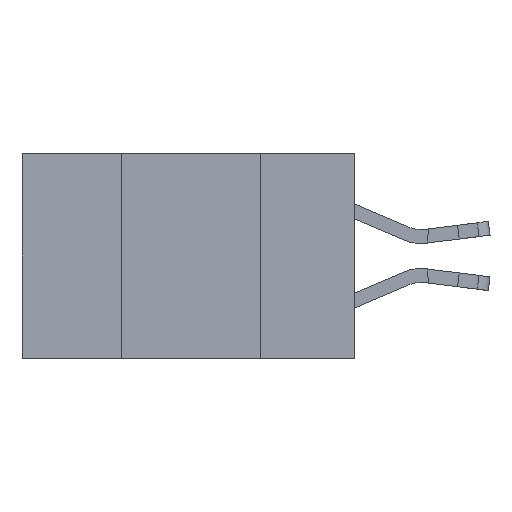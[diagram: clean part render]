
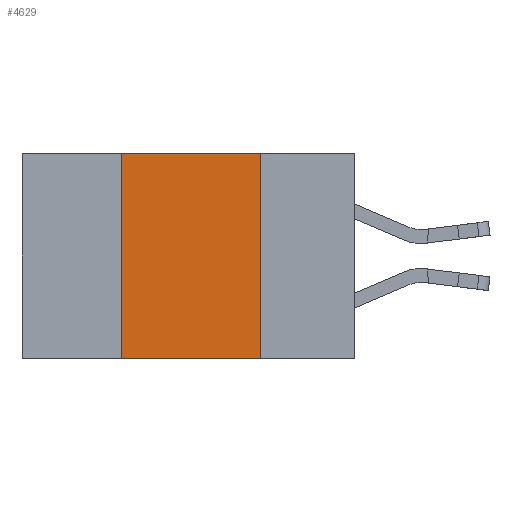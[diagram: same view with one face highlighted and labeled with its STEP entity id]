
A CAD part, left-side view. The second image highlights one B-rep face of the part: STEP entity #4629.
In plain terms, the highlighted planar face has unit normal (-1, 0, 0).
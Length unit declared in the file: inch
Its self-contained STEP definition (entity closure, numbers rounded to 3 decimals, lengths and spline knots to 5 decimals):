
#90 = CARTESIAN_POINT ( 'NONE',  ( 0., 0.17, 0. ) ) ;
#99 = DIRECTION ( 'NONE',  ( 1., 0., 0. ) ) ;
#483 = EDGE_CURVE ( 'NONE', #2353, #5029, #673, .T. ) ;
#532 = ORIENTED_EDGE ( 'NONE', *, *, #12385, .T. ) ;
#673 = LINE ( 'NONE', #90, #5557 ) ;
#1401 = CARTESIAN_POINT ( 'NONE',  ( 0., 0.42, 0. ) ) ;
#1446 = LINE ( 'NONE', #12028, #9452 ) ;
#2353 = VERTEX_POINT ( 'NONE', #11768 ) ;
#3140 = EDGE_LOOP ( 'NONE', ( #6022, #5442, #12497, #532 ) ) ;
#3511 = VECTOR ( 'NONE', #8682, 39.37008 ) ;
#4629 = ADVANCED_FACE ( 'NONE', ( #11145 ), #12619, .F. ) ;
#4881 = VECTOR ( 'NONE', #6036, 39.37008 ) ;
#5029 = VERTEX_POINT ( 'NONE', #9096 ) ;
#5442 = ORIENTED_EDGE ( 'NONE', *, *, #11890, .F. ) ;
#5557 = VECTOR ( 'NONE', #11538, 39.37008 ) ;
#5759 = DIRECTION ( 'NONE',  ( 0., -1., 0. ) ) ;
#6022 = ORIENTED_EDGE ( 'NONE', *, *, #483, .F. ) ;
#6036 = DIRECTION ( 'NONE',  ( 0., -1., 0. ) ) ;
#6529 = CARTESIAN_POINT ( 'NONE',  ( 0., 0.42, 0. ) ) ;
#6677 = CARTESIAN_POINT ( 'NONE',  ( 0., 0.42, -0.37 ) ) ;
#6763 = EDGE_CURVE ( 'NONE', #12288, #7881, #11179, .T. ) ;
#7321 = LINE ( 'NONE', #12318, #4881 ) ;
#7367 = DIRECTION ( 'NONE',  ( 0., 0., -1. ) ) ;
#7881 = VERTEX_POINT ( 'NONE', #6529 ) ;
#8682 = DIRECTION ( 'NONE',  ( 0., 0., 1. ) ) ;
#9096 = CARTESIAN_POINT ( 'NONE',  ( 0., 0.17, -0.37 ) ) ;
#9452 = VECTOR ( 'NONE', #5759, 39.37008 ) ;
#10648 = AXIS2_PLACEMENT_3D ( 'NONE', #11546, #99, #7367 ) ;
#11145 = FACE_OUTER_BOUND ( 'NONE', #3140, .T. ) ;
#11179 = LINE ( 'NONE', #1401, #3511 ) ;
#11538 = DIRECTION ( 'NONE',  ( 0., 0., -1. ) ) ;
#11546 = CARTESIAN_POINT ( 'NONE',  ( 0., 0.6, 0. ) ) ;
#11768 = CARTESIAN_POINT ( 'NONE',  ( 0., 0.17, 0. ) ) ;
#11890 = EDGE_CURVE ( 'NONE', #7881, #2353, #7321, .T. ) ;
#12028 = CARTESIAN_POINT ( 'NONE',  ( 0., 0.6, -0.37 ) ) ;
#12288 = VERTEX_POINT ( 'NONE', #6677 ) ;
#12318 = CARTESIAN_POINT ( 'NONE',  ( 0., 0.6, 0. ) ) ;
#12385 = EDGE_CURVE ( 'NONE', #12288, #5029, #1446, .T. ) ;
#12497 = ORIENTED_EDGE ( 'NONE', *, *, #6763, .F. ) ;
#12619 = PLANE ( 'NONE',  #10648 ) ;
